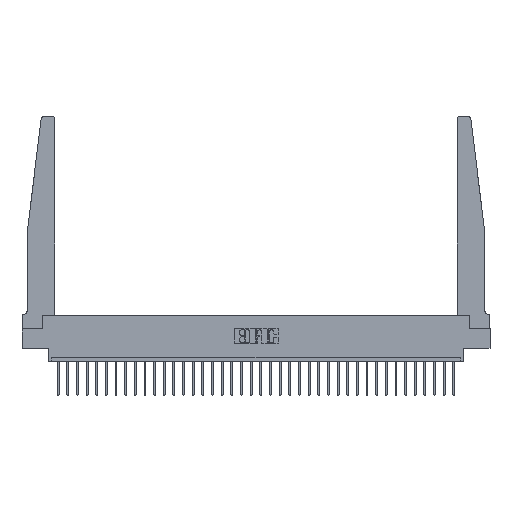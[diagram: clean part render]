
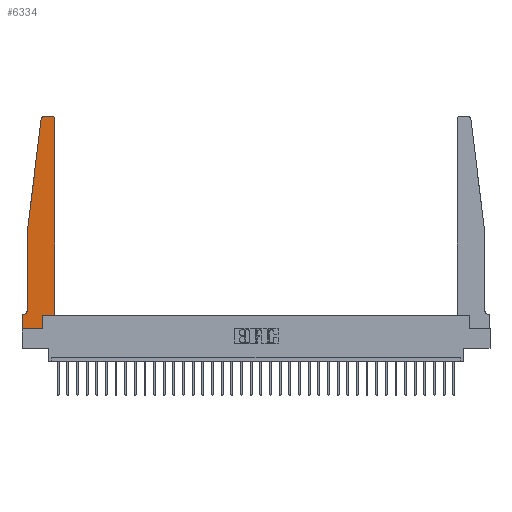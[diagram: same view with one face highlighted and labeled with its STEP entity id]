
A CAD part, top view. The second image highlights one B-rep face of the part: STEP entity #6334.
In plain terms, the highlighted planar face has unit normal (0, 0, 1).
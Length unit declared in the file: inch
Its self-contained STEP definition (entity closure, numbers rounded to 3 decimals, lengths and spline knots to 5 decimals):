
#145 = CARTESIAN_POINT ( 'NONE',  ( 0., 0., 0.37 ) ) ;
#275 = LINE ( 'NONE', #25989, #15969 ) ;
#640 = VERTEX_POINT ( 'NONE', #16409 ) ;
#773 = LINE ( 'NONE', #3751, #22465 ) ;
#1964 = DIRECTION ( 'NONE',  ( 0., 1., 0. ) ) ;
#2113 = CARTESIAN_POINT ( 'NONE',  ( 0.27653, 2.72, 0.37 ) ) ;
#2554 = CARTESIAN_POINT ( 'NONE',  ( 0.395, 2.75, 0.37 ) ) ;
#2906 = EDGE_CURVE ( 'NONE', #28950, #15022, #30398, .T. ) ;
#3019 = EDGE_CURVE ( 'NONE', #28087, #11537, #3861, .T. ) ;
#3538 = DIRECTION ( 'NONE',  ( 0., -1., 0. ) ) ;
#3561 = LINE ( 'NONE', #28855, #17764 ) ;
#3668 = CARTESIAN_POINT ( 'NONE',  ( 0.065, 0.1875, 0.37 ) ) ;
#3751 = CARTESIAN_POINT ( 'NONE',  ( 0.065, 1.25, 0.37 ) ) ;
#3799 = CARTESIAN_POINT ( 'NONE',  ( 0.25, 2.75, 0.37 ) ) ;
#3861 = LINE ( 'NONE', #3799, #8264 ) ;
#4489 = AXIS2_PLACEMENT_3D ( 'NONE', #11596, #28171, #13619 ) ;
#5279 = VERTEX_POINT ( 'NONE', #21258 ) ;
#5408 = VECTOR ( 'NONE', #26610, 39.37008 ) ;
#5459 = DIRECTION ( 'NONE',  ( 1., 0., 0. ) ) ;
#5623 = ORIENTED_EDGE ( 'NONE', *, *, #11284, .T. ) ;
#5950 = VECTOR ( 'NONE', #8668, 39.37008 ) ;
#6084 = DIRECTION ( 'NONE',  ( -1., 0., 0. ) ) ;
#6334 = ADVANCED_FACE ( 'NONE', ( #16313 ), #11921, .T. ) ;
#6899 = DIRECTION ( 'NONE',  ( 0., 0., 1. ) ) ;
#7271 = VECTOR ( 'NONE', #17969, 39.37008 ) ;
#7613 = ORIENTED_EDGE ( 'NONE', *, *, #23480, .T. ) ;
#8229 = DIRECTION ( 'NONE',  ( 0., 0., 1. ) ) ;
#8264 = VECTOR ( 'NONE', #6084, 39.37008 ) ;
#8365 = CARTESIAN_POINT ( 'NONE',  ( 0.065, 1.25, 0.37 ) ) ;
#8446 = VERTEX_POINT ( 'NONE', #24218 ) ;
#8668 = DIRECTION ( 'NONE',  ( -0.122, -0.992, 0. ) ) ;
#9274 = EDGE_CURVE ( 'NONE', #11537, #8446, #11690, .T. ) ;
#9656 = ORIENTED_EDGE ( 'NONE', *, *, #25469, .T. ) ;
#10481 = VECTOR ( 'NONE', #16938, 39.37008 ) ;
#11274 = EDGE_CURVE ( 'NONE', #16150, #15650, #25626, .T. ) ;
#11284 = EDGE_CURVE ( 'NONE', #640, #28950, #3561, .T. ) ;
#11537 = VERTEX_POINT ( 'NONE', #14897 ) ;
#11596 = CARTESIAN_POINT ( 'NONE',  ( 0.015, 0.2375, 0.37 ) ) ;
#11690 = CIRCLE ( 'NONE', #14967, 0.03 ) ;
#11910 = EDGE_CURVE ( 'NONE', #15868, #16150, #19994, .T. ) ;
#11911 = CIRCLE ( 'NONE', #26304, 0.03 ) ;
#11921 = PLANE ( 'NONE',  #21570 ) ;
#12232 = DIRECTION ( 'NONE',  ( 1., 0., 0. ) ) ;
#12516 = CARTESIAN_POINT ( 'NONE',  ( 0.425, 0.18, 0.37 ) ) ;
#12978 = ORIENTED_EDGE ( 'NONE', *, *, #3019, .T. ) ;
#13619 = DIRECTION ( 'NONE',  ( -1., 0., 0. ) ) ;
#14107 = ORIENTED_EDGE ( 'NONE', *, *, #11274, .T. ) ;
#14189 = CARTESIAN_POINT ( 'NONE',  ( 0.425, 2.72, 0.37 ) ) ;
#14417 = EDGE_CURVE ( 'NONE', #23471, #15868, #25840, .T. ) ;
#14633 = CARTESIAN_POINT ( 'NONE',  ( 0.015, 0.1875, 0.37 ) ) ;
#14639 = CARTESIAN_POINT ( 'NONE',  ( 0.425, 0.18, 0.37 ) ) ;
#14682 = EDGE_CURVE ( 'NONE', #15022, #28087, #11911, .T. ) ;
#14897 = CARTESIAN_POINT ( 'NONE',  ( 0.27653, 2.75, 0.37 ) ) ;
#14967 = AXIS2_PLACEMENT_3D ( 'NONE', #2113, #6899, #23313 ) ;
#15022 = VERTEX_POINT ( 'NONE', #14189 ) ;
#15266 = CARTESIAN_POINT ( 'NONE',  ( 0.395, 2.72, 0.37 ) ) ;
#15594 = ORIENTED_EDGE ( 'NONE', *, *, #14417, .T. ) ;
#15650 = VERTEX_POINT ( 'NONE', #25399 ) ;
#15868 = VERTEX_POINT ( 'NONE', #14633 ) ;
#15969 = VECTOR ( 'NONE', #1964, 39.37008 ) ;
#16150 = VERTEX_POINT ( 'NONE', #18588 ) ;
#16313 = FACE_OUTER_BOUND ( 'NONE', #20375, .T. ) ;
#16409 = CARTESIAN_POINT ( 'NONE',  ( 0.2605, 0.18, 0.37 ) ) ;
#16938 = DIRECTION ( 'NONE',  ( 0., 1., 0. ) ) ;
#16952 = DIRECTION ( 'NONE',  ( 1., 0., 0. ) ) ;
#17281 = VERTEX_POINT ( 'NONE', #30594 ) ;
#17384 = ORIENTED_EDGE ( 'NONE', *, *, #14682, .T. ) ;
#17457 = EDGE_CURVE ( 'NONE', #8446, #5279, #23520, .T. ) ;
#17764 = VECTOR ( 'NONE', #12232, 39.37008 ) ;
#17969 = DIRECTION ( 'NONE',  ( -1., 0., 0. ) ) ;
#18046 = VECTOR ( 'NONE', #16952, 39.37008 ) ;
#18588 = CARTESIAN_POINT ( 'NONE',  ( 0., 0.1875, 0.37 ) ) ;
#19929 = DIRECTION ( 'NONE',  ( 0., 0., 1. ) ) ;
#19994 = LINE ( 'NONE', #3668, #7271 ) ;
#20220 = ORIENTED_EDGE ( 'NONE', *, *, #11910, .T. ) ;
#20375 = EDGE_LOOP ( 'NONE', ( #12978, #26976, #30300, #7613, #15594, #20220, #14107, #28203, #9656, #5623, #25070, #17384 ) ) ;
#21258 = CARTESIAN_POINT ( 'NONE',  ( 0.065, 1.25, 0.37 ) ) ;
#21570 = AXIS2_PLACEMENT_3D ( 'NONE', #26910, #19929, #29555 ) ;
#21652 = CARTESIAN_POINT ( 'NONE',  ( 0., 0., 0.37 ) ) ;
#22465 = VECTOR ( 'NONE', #3538, 39.37008 ) ;
#23313 = DIRECTION ( 'NONE',  ( 1., 0., 0. ) ) ;
#23471 = VERTEX_POINT ( 'NONE', #29997 ) ;
#23480 = EDGE_CURVE ( 'NONE', #5279, #23471, #773, .T. ) ;
#23520 = LINE ( 'NONE', #8365, #5950 ) ;
#24218 = CARTESIAN_POINT ( 'NONE',  ( 0.24675, 2.72367, 0.37 ) ) ;
#25070 = ORIENTED_EDGE ( 'NONE', *, *, #2906, .T. ) ;
#25399 = CARTESIAN_POINT ( 'NONE',  ( 0., 0., 0.37 ) ) ;
#25469 = EDGE_CURVE ( 'NONE', #17281, #640, #275, .T. ) ;
#25626 = LINE ( 'NONE', #21652, #5408 ) ;
#25840 = CIRCLE ( 'NONE', #4489, 0.05 ) ;
#25899 = LINE ( 'NONE', #145, #18046 ) ;
#25989 = CARTESIAN_POINT ( 'NONE',  ( 0.2605, 0.18, 0.37 ) ) ;
#26304 = AXIS2_PLACEMENT_3D ( 'NONE', #15266, #8229, #5459 ) ;
#26610 = DIRECTION ( 'NONE',  ( 0., -1., 0. ) ) ;
#26910 = CARTESIAN_POINT ( 'NONE',  ( 0., 0.1875, 0.37 ) ) ;
#26976 = ORIENTED_EDGE ( 'NONE', *, *, #9274, .T. ) ;
#28042 = EDGE_CURVE ( 'NONE', #15650, #17281, #25899, .T. ) ;
#28087 = VERTEX_POINT ( 'NONE', #2554 ) ;
#28171 = DIRECTION ( 'NONE',  ( 0., 0., -1. ) ) ;
#28203 = ORIENTED_EDGE ( 'NONE', *, *, #28042, .T. ) ;
#28855 = CARTESIAN_POINT ( 'NONE',  ( 0.425, 0.18, 0.37 ) ) ;
#28950 = VERTEX_POINT ( 'NONE', #12516 ) ;
#29555 = DIRECTION ( 'NONE',  ( 1., 0., 0. ) ) ;
#29997 = CARTESIAN_POINT ( 'NONE',  ( 0.065, 0.2375, 0.37 ) ) ;
#30300 = ORIENTED_EDGE ( 'NONE', *, *, #17457, .T. ) ;
#30398 = LINE ( 'NONE', #14639, #10481 ) ;
#30594 = CARTESIAN_POINT ( 'NONE',  ( 0.2605, 0., 0.37 ) ) ;
